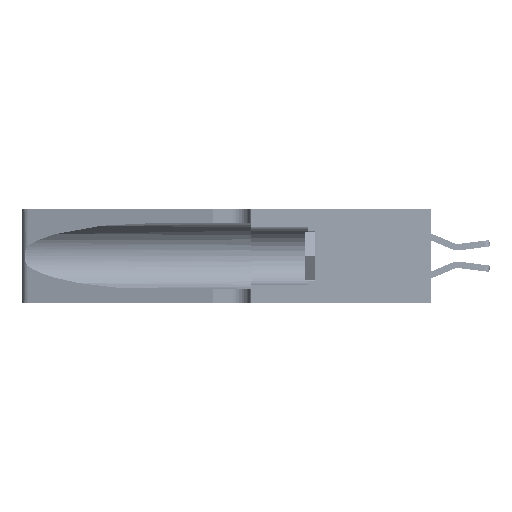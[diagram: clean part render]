
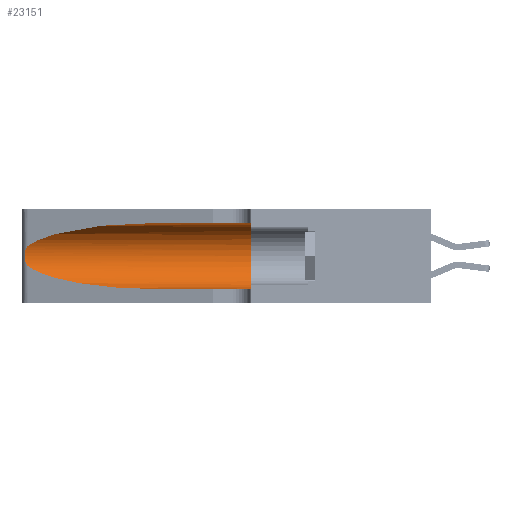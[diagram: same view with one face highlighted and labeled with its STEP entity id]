
A CAD part, left-side view. The second image highlights one B-rep face of the part: STEP entity #23151.
In plain terms, the highlighted cylindrical face has radius 3.308 mm (diameter 6.617 mm), a partial arc.
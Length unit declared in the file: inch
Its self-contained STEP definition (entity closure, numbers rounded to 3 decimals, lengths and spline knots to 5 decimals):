
#476 = VERTEX_POINT ( 'NONE', #32982 ) ;
#567 = CARTESIAN_POINT ( 'NONE',  ( 0.25487, 1.22718, 0.22369 ) ) ;
#702 = CARTESIAN_POINT ( 'NONE',  ( 0.25487, 1.22718, 0.14631 ) ) ;
#738 = CARTESIAN_POINT ( 'NONE',  ( 0.25639, 1.23186, 0.15144 ) ) ;
#958 = ORIENTED_EDGE ( 'NONE', *, *, #4290, .F. ) ;
#2128 = CARTESIAN_POINT ( 'NONE',  ( 0.2373, 1.15595, 0.08982 ) ) ;
#2579 = CIRCLE ( 'NONE', #20330, 0.13025 ) ;
#4270 = ORIENTED_EDGE ( 'NONE', *, *, #9829, .F. ) ;
#4290 = EDGE_CURVE ( 'NONE', #24728, #44372, #17180, .T. ) ;
#4506 = CARTESIAN_POINT ( 'NONE',  ( 0.1305, 0.35, 0.31525 ) ) ;
#4894 = CARTESIAN_POINT ( 'NONE',  ( 0.25487, 1.22718, 0.14631 ) ) ;
#6779 =( BOUNDED_CURVE ( )  B_SPLINE_CURVE ( 3, ( #18650, #2128, #51449, #26962 ),
 .UNSPECIFIED., .F., .F. ) 
 B_SPLINE_CURVE_WITH_KNOTS ( ( 4, 4 ),
 ( 3.44316, 4.71239 ),
 .UNSPECIFIED. ) 
 CURVE ( )  GEOMETRIC_REPRESENTATION_ITEM ( )  RATIONAL_B_SPLINE_CURVE ( ( 1., 0.87, 0.87, 1. ) ) 
 REPRESENTATION_ITEM ( '' )  );
#6919 = CARTESIAN_POINT ( 'NONE',  ( 0.1305, 1.61858, 0.185 ) ) ;
#8131 =( BOUNDED_CURVE ( )  B_SPLINE_CURVE ( 3, ( #13842, #34284, #30192, #17964 ),
 .UNSPECIFIED., .F., .T. ) 
 B_SPLINE_CURVE_WITH_KNOTS ( ( 4, 4 ),
 ( 1.5708, 2.84003 ),
 .UNSPECIFIED. ) 
 CURVE ( )  GEOMETRIC_REPRESENTATION_ITEM ( )  RATIONAL_B_SPLINE_CURVE ( ( 1., 0.87, 0.87, 1. ) ) 
 REPRESENTATION_ITEM ( '' )  );
#8844 = CARTESIAN_POINT ( 'NONE',  ( 0.25639, 1.23184, 0.21858 ) ) ;
#9829 = EDGE_CURVE ( 'NONE', #44372, #476, #2579, .T. ) ;
#10167 = EDGE_CURVE ( 'NONE', #24728, #29264, #8131, .T. ) ;
#10296 = VECTOR ( 'NONE', #44682, 39.37008 ) ;
#12973 = CARTESIAN_POINT ( 'NONE',  ( 0.25854, 1.2359, 0.20912 ) ) ;
#13842 = CARTESIAN_POINT ( 'NONE',  ( 0.1305, 0.72297, 0.31525 ) ) ;
#14367 = AXIS2_PLACEMENT_3D ( 'NONE', #6919, #19286, #47970 ) ;
#16044 = DIRECTION ( 'NONE',  ( 0., 1., 0. ) ) ;
#17092 = CARTESIAN_POINT ( 'NONE',  ( 0.26075, 1.23896, 0.19203 ) ) ;
#17180 = LINE ( 'NONE', #22506, #51201 ) ;
#17751 = EDGE_CURVE ( 'NONE', #29264, #33226, #27536, .T. ) ;
#17964 = CARTESIAN_POINT ( 'NONE',  ( 0.25487, 1.22718, 0.22369 ) ) ;
#18650 = CARTESIAN_POINT ( 'NONE',  ( 0.25487, 1.22718, 0.14631 ) ) ;
#18845 = ORIENTED_EDGE ( 'NONE', *, *, #33467, .T. ) ;
#19286 = DIRECTION ( 'NONE',  ( 0., -1., 0. ) ) ;
#20330 = AXIS2_PLACEMENT_3D ( 'NONE', #40574, #16044, #44716 ) ;
#21248 = LINE ( 'NONE', #40545, #10296 ) ;
#21259 = CARTESIAN_POINT ( 'NONE',  ( 0.26017, 1.23833, 0.17102 ) ) ;
#22506 = CARTESIAN_POINT ( 'NONE',  ( 0.1305, 1.61858, 0.31525 ) ) ;
#22981 = CARTESIAN_POINT ( 'NONE',  ( 0.25487, 1.22718, 0.22369 ) ) ;
#23151 = ADVANCED_FACE ( 'NONE', ( #47728 ), #24667, .F. ) ;
#23694 = ORIENTED_EDGE ( 'NONE', *, *, #33047, .T. ) ;
#24667 = CYLINDRICAL_SURFACE ( 'NONE', #14367, 0.13025 ) ;
#24728 = VERTEX_POINT ( 'NONE', #35691 ) ;
#25397 = CARTESIAN_POINT ( 'NONE',  ( 0.25789, 1.23486, 0.15765 ) ) ;
#26962 = CARTESIAN_POINT ( 'NONE',  ( 0.1305, 0.72297, 0.05475 ) ) ;
#27536 = B_SPLINE_CURVE_WITH_KNOTS ( 'NONE', 3,
 ( #567, #41474, #8844, #37520, #12973, #41663, #17092, #45791, #21259, #49912, #25397, #738, #29506, #4894 ),
 .UNSPECIFIED., .F., .F.,
 ( 4, 2, 2, 2, 2, 2, 4 ),
 ( 0., 0.00027, 0.00053, 0.00107, 0.0016, 0.00187, 0.00214 ),
 .UNSPECIFIED. ) ;
#29264 = VERTEX_POINT ( 'NONE', #22981 ) ;
#29506 = CARTESIAN_POINT ( 'NONE',  ( 0.25555, 1.22993, 0.14849 ) ) ;
#30192 = CARTESIAN_POINT ( 'NONE',  ( 0.2373, 1.15595, 0.28018 ) ) ;
#32982 = CARTESIAN_POINT ( 'NONE',  ( 0.1305, 0.35, 0.05475 ) ) ;
#33047 = EDGE_CURVE ( 'NONE', #34992, #476, #21248, .T. ) ;
#33226 = VERTEX_POINT ( 'NONE', #702 ) ;
#33467 = EDGE_CURVE ( 'NONE', #33226, #34992, #6779, .T. ) ;
#34284 = CARTESIAN_POINT ( 'NONE',  ( 0.18966, 0.96281, 0.31525 ) ) ;
#34992 = VERTEX_POINT ( 'NONE', #40185 ) ;
#35691 = CARTESIAN_POINT ( 'NONE',  ( 0.1305, 0.72297, 0.31525 ) ) ;
#37520 = CARTESIAN_POINT ( 'NONE',  ( 0.25787, 1.23484, 0.2124 ) ) ;
#40185 = CARTESIAN_POINT ( 'NONE',  ( 0.1305, 0.72297, 0.05475 ) ) ;
#40545 = CARTESIAN_POINT ( 'NONE',  ( 0.1305, 1.61858, 0.05475 ) ) ;
#40574 = CARTESIAN_POINT ( 'NONE',  ( 0.1305, 0.35, 0.185 ) ) ;
#41474 = CARTESIAN_POINT ( 'NONE',  ( 0.25555, 1.22994, 0.2215 ) ) ;
#41663 = CARTESIAN_POINT ( 'NONE',  ( 0.26018, 1.23835, 0.19895 ) ) ;
#44372 = VERTEX_POINT ( 'NONE', #4506 ) ;
#44682 = DIRECTION ( 'NONE',  ( 0., -1., 0. ) ) ;
#44716 = DIRECTION ( 'NONE',  ( 0., 0., 1. ) ) ;
#44828 = EDGE_LOOP ( 'NONE', ( #46961, #50507, #18845, #23694, #4270, #958 ) ) ;
#45791 = CARTESIAN_POINT ( 'NONE',  ( 0.26075, 1.23896, 0.178 ) ) ;
#46961 = ORIENTED_EDGE ( 'NONE', *, *, #10167, .T. ) ;
#47728 = FACE_OUTER_BOUND ( 'NONE', #44828, .T. ) ;
#47970 = DIRECTION ( 'NONE',  ( 0., 0., -1. ) ) ;
#49912 = CARTESIAN_POINT ( 'NONE',  ( 0.25856, 1.23593, 0.16098 ) ) ;
#50507 = ORIENTED_EDGE ( 'NONE', *, *, #17751, .T. ) ;
#51145 = DIRECTION ( 'NONE',  ( 0., -1., 0. ) ) ;
#51201 = VECTOR ( 'NONE', #51145, 39.37008 ) ;
#51449 = CARTESIAN_POINT ( 'NONE',  ( 0.18966, 0.96281, 0.05475 ) ) ;
